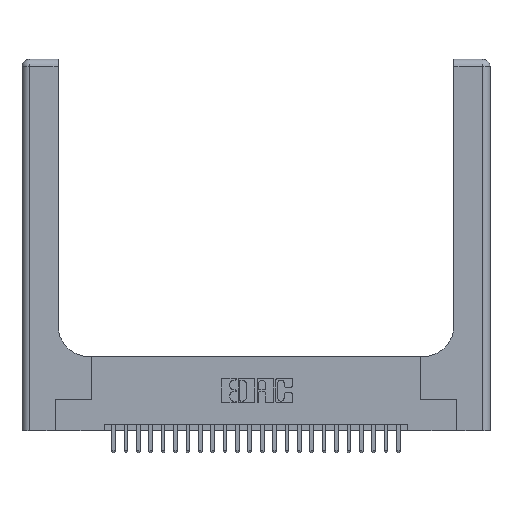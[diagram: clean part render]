
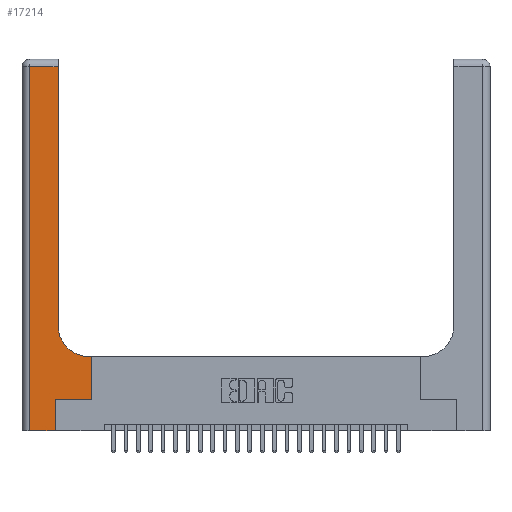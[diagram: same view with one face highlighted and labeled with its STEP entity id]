
A CAD part, top view. The second image highlights one B-rep face of the part: STEP entity #17214.
In plain terms, the highlighted planar face has unit normal (0, 0, 1).
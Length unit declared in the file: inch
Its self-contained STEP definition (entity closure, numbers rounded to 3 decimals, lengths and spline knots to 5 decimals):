
#683 = DIRECTION ( 'NONE',  ( 0., 0., -1. ) ) ;
#824 = ORIENTED_EDGE ( 'NONE', *, *, #5557, .T. ) ;
#887 = ORIENTED_EDGE ( 'NONE', *, *, #10690, .T. ) ;
#1107 = ORIENTED_EDGE ( 'NONE', *, *, #17530, .T. ) ;
#1203 = VERTEX_POINT ( 'NONE', #20380 ) ;
#1395 = CARTESIAN_POINT ( 'NONE',  ( 0.06, 3., 0.37 ) ) ;
#1678 = CARTESIAN_POINT ( 'NONE',  ( 0.5585, 0.6, 0.37 ) ) ;
#1705 = DIRECTION ( 'NONE',  ( -1., 0., 0. ) ) ;
#2388 = VERTEX_POINT ( 'NONE', #1678 ) ;
#2467 = LINE ( 'NONE', #24038, #7319 ) ;
#2578 = VERTEX_POINT ( 'NONE', #23510 ) ;
#3403 = ORIENTED_EDGE ( 'NONE', *, *, #7503, .T. ) ;
#3712 = CARTESIAN_POINT ( 'NONE',  ( 0.269, 0., 0.37 ) ) ;
#3878 = AXIS2_PLACEMENT_3D ( 'NONE', #23859, #11655, #25866 ) ;
#4126 = ORIENTED_EDGE ( 'NONE', *, *, #17624, .T. ) ;
#4319 = DIRECTION ( 'NONE',  ( 0., 1., 0. ) ) ;
#4610 = CARTESIAN_POINT ( 'NONE',  ( 0.5585, 0.25, 0.37 ) ) ;
#4676 = DIRECTION ( 'NONE',  ( 1., 0., 0. ) ) ;
#5521 = FACE_OUTER_BOUND ( 'NONE', #12542, .T. ) ;
#5557 = EDGE_CURVE ( 'NONE', #18674, #10101, #8265, .T. ) ;
#5820 = CARTESIAN_POINT ( 'NONE',  ( 0., 0., 0.37 ) ) ;
#6703 = DIRECTION ( 'NONE',  ( 0., 1., 0. ) ) ;
#7162 = AXIS2_PLACEMENT_3D ( 'NONE', #13076, #683, #15172 ) ;
#7319 = VECTOR ( 'NONE', #13995, 39.37008 ) ;
#7499 = PLANE ( 'NONE',  #3878 ) ;
#7503 = EDGE_CURVE ( 'NONE', #22070, #13257, #24474, .T. ) ;
#7775 = ORIENTED_EDGE ( 'NONE', *, *, #11536, .T. ) ;
#7967 = VECTOR ( 'NONE', #18243, 39.37008 ) ;
#8265 = LINE ( 'NONE', #5820, #23934 ) ;
#8484 = CARTESIAN_POINT ( 'NONE',  ( 0.2915, 3., 0.37 ) ) ;
#8824 = VECTOR ( 'NONE', #23602, 39.37008 ) ;
#10101 = VERTEX_POINT ( 'NONE', #3712 ) ;
#10358 = VECTOR ( 'NONE', #4676, 39.37008 ) ;
#10636 = ORIENTED_EDGE ( 'NONE', *, *, #18961, .T. ) ;
#10690 = EDGE_CURVE ( 'NONE', #2388, #2578, #18741, .T. ) ;
#11002 = LINE ( 'NONE', #23067, #10358 ) ;
#11394 = CARTESIAN_POINT ( 'NONE',  ( 0., 2.94, 0.37 ) ) ;
#11536 = EDGE_CURVE ( 'NONE', #2578, #21901, #25944, .T. ) ;
#11655 = DIRECTION ( 'NONE',  ( 0., 0., -1. ) ) ;
#12542 = EDGE_LOOP ( 'NONE', ( #1107, #3403, #20231, #824, #13198, #4126, #10636, #887, #7775 ) ) ;
#12663 = VECTOR ( 'NONE', #1705, 39.37008 ) ;
#12914 = VECTOR ( 'NONE', #4319, 39.37008 ) ;
#13076 = CARTESIAN_POINT ( 'NONE',  ( 0.5415, 0.85, 0.37 ) ) ;
#13198 = ORIENTED_EDGE ( 'NONE', *, *, #13672, .T. ) ;
#13257 = VERTEX_POINT ( 'NONE', #18931 ) ;
#13672 = EDGE_CURVE ( 'NONE', #10101, #19598, #2467, .T. ) ;
#13995 = DIRECTION ( 'NONE',  ( 0., 1., 0. ) ) ;
#15172 = DIRECTION ( 'NONE',  ( 1., 0., 0. ) ) ;
#16925 = CARTESIAN_POINT ( 'NONE',  ( 0.269, 0.25, 0.37 ) ) ;
#17111 = CARTESIAN_POINT ( 'NONE',  ( 0.2915, 0.85, 0.37 ) ) ;
#17214 = ADVANCED_FACE ( 'NONE', ( #5521 ), #7499, .F. ) ;
#17530 = EDGE_CURVE ( 'NONE', #21901, #22070, #19656, .T. ) ;
#17624 = EDGE_CURVE ( 'NONE', #19598, #1203, #11002, .T. ) ;
#18243 = DIRECTION ( 'NONE',  ( 0., -1., 0. ) ) ;
#18302 = VECTOR ( 'NONE', #6703, 39.37008 ) ;
#18674 = VERTEX_POINT ( 'NONE', #24234 ) ;
#18741 = LINE ( 'NONE', #26197, #12663 ) ;
#18931 = CARTESIAN_POINT ( 'NONE',  ( 0.06, 2.94, 0.37 ) ) ;
#18961 = EDGE_CURVE ( 'NONE', #1203, #2388, #24324, .T. ) ;
#19598 = VERTEX_POINT ( 'NONE', #16925 ) ;
#19656 = LINE ( 'NONE', #8484, #12914 ) ;
#19679 = CARTESIAN_POINT ( 'NONE',  ( 0.2915, 2.94, 0.37 ) ) ;
#19907 = EDGE_CURVE ( 'NONE', #13257, #18674, #24899, .T. ) ;
#20231 = ORIENTED_EDGE ( 'NONE', *, *, #19907, .T. ) ;
#20380 = CARTESIAN_POINT ( 'NONE',  ( 0.5585, 0.25, 0.37 ) ) ;
#21901 = VERTEX_POINT ( 'NONE', #17111 ) ;
#22070 = VERTEX_POINT ( 'NONE', #19679 ) ;
#22220 = DIRECTION ( 'NONE',  ( 1., 0., 0. ) ) ;
#23067 = CARTESIAN_POINT ( 'NONE',  ( 0.269, 0.25, 0.37 ) ) ;
#23510 = CARTESIAN_POINT ( 'NONE',  ( 0.5415, 0.6, 0.37 ) ) ;
#23602 = DIRECTION ( 'NONE',  ( -1., 0., 0. ) ) ;
#23859 = CARTESIAN_POINT ( 'NONE',  ( 0., 3., 0.37 ) ) ;
#23934 = VECTOR ( 'NONE', #22220, 39.37008 ) ;
#24038 = CARTESIAN_POINT ( 'NONE',  ( 0.269, 0., 0.37 ) ) ;
#24234 = CARTESIAN_POINT ( 'NONE',  ( 0.06, 0., 0.37 ) ) ;
#24324 = LINE ( 'NONE', #4610, #18302 ) ;
#24474 = LINE ( 'NONE', #11394, #8824 ) ;
#24899 = LINE ( 'NONE', #1395, #7967 ) ;
#25866 = DIRECTION ( 'NONE',  ( -1., 0., 0. ) ) ;
#25944 = CIRCLE ( 'NONE', #7162, 0.25 ) ;
#26197 = CARTESIAN_POINT ( 'NONE',  ( 0.2915, 0.6, 0.37 ) ) ;
